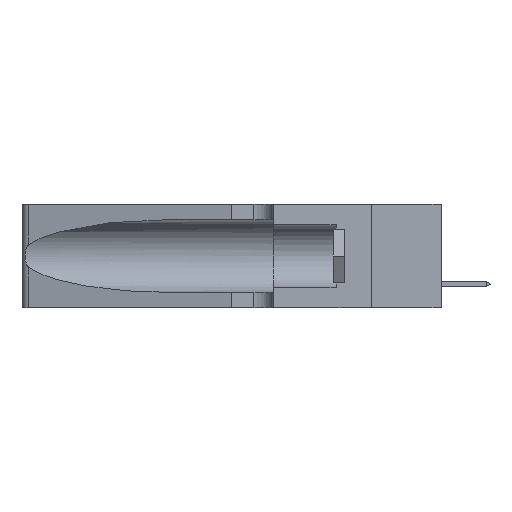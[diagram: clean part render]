
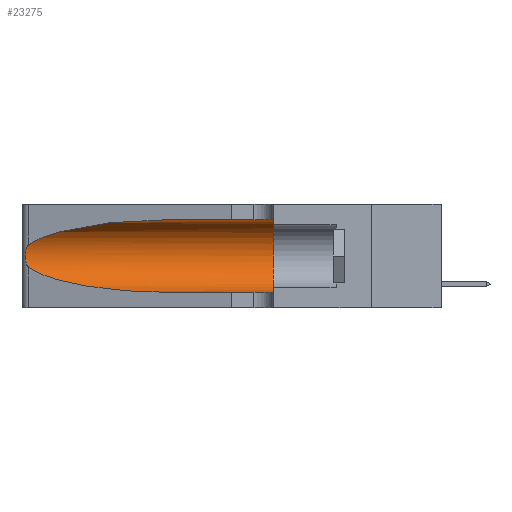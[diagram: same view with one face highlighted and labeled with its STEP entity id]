
A CAD part, left-side view. The second image highlights one B-rep face of the part: STEP entity #23275.
In plain terms, the highlighted cylindrical face has radius 3.308 mm (diameter 6.617 mm), a partial arc.
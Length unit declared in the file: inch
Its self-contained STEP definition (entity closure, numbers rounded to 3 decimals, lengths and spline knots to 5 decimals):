
#220 = CARTESIAN_POINT ( 'NONE',  ( 0.1305, 1.61858, 0.185 ) ) ;
#296 = CARTESIAN_POINT ( 'NONE',  ( 0.25555, 1.22993, 0.14849 ) ) ;
#635 = CIRCLE ( 'NONE', #13194, 0.13025 ) ;
#764 = CARTESIAN_POINT ( 'NONE',  ( 0.1305, 0.72297, 0.05475 ) ) ;
#858 = CARTESIAN_POINT ( 'NONE',  ( 0.1305, 0.72297, 0.31525 ) ) ;
#1042 = DIRECTION ( 'NONE',  ( 0., 0., 1. ) ) ;
#2047 = AXIS2_PLACEMENT_3D ( 'NONE', #220, #3992, #23539 ) ;
#2331 = CARTESIAN_POINT ( 'NONE',  ( 0.25639, 1.23186, 0.15144 ) ) ;
#2939 = VERTEX_POINT ( 'NONE', #21987 ) ;
#3081 = VECTOR ( 'NONE', #9644, 39.37008 ) ;
#3137 = LINE ( 'NONE', #10759, #8001 ) ;
#3707 = CYLINDRICAL_SURFACE ( 'NONE', #2047, 0.13025 ) ;
#3813 = VERTEX_POINT ( 'NONE', #22875 ) ;
#3992 = DIRECTION ( 'NONE',  ( 0., -1., 0. ) ) ;
#4366 = CARTESIAN_POINT ( 'NONE',  ( 0.25789, 1.23486, 0.15765 ) ) ;
#4526 = CARTESIAN_POINT ( 'NONE',  ( 0.2373, 1.15595, 0.08982 ) ) ;
#4982 = DIRECTION ( 'NONE',  ( 0., -1., 0. ) ) ;
#6987 = VERTEX_POINT ( 'NONE', #23021 ) ;
#7429 = ORIENTED_EDGE ( 'NONE', *, *, #23166, .T. ) ;
#7462 = CARTESIAN_POINT ( 'NONE',  ( 0.25487, 1.22718, 0.22369 ) ) ;
#7702 = CARTESIAN_POINT ( 'NONE',  ( 0.25555, 1.22994, 0.2215 ) ) ;
#8001 = VECTOR ( 'NONE', #4982, 39.37008 ) ;
#9298 = CARTESIAN_POINT ( 'NONE',  ( 0.1305, 1.61858, 0.05475 ) ) ;
#9644 = DIRECTION ( 'NONE',  ( 0., -1., 0. ) ) ;
#9649 = EDGE_CURVE ( 'NONE', #6987, #13313, #10922, .T. ) ;
#9994 = CARTESIAN_POINT ( 'NONE',  ( 0.25487, 1.22718, 0.22369 ) ) ;
#10265 = CARTESIAN_POINT ( 'NONE',  ( 0.25487, 1.22718, 0.14631 ) ) ;
#10544 = CARTESIAN_POINT ( 'NONE',  ( 0.25487, 1.22718, 0.14631 ) ) ;
#10554 = CARTESIAN_POINT ( 'NONE',  ( 0.26018, 1.23835, 0.19895 ) ) ;
#10759 = CARTESIAN_POINT ( 'NONE',  ( 0.1305, 1.61858, 0.31525 ) ) ;
#10922 = B_SPLINE_CURVE_WITH_KNOTS ( 'NONE', 3,
 ( #7462, #7702, #11607, #17518, #19937, #10554, #22678, #18509, #24903, #15710, #4366, #2331, #296, #10265 ),
 .UNSPECIFIED., .F., .F.,
 ( 4, 2, 2, 2, 2, 2, 4 ),
 ( 0., 0.00027, 0.00053, 0.00107, 0.0016, 0.00187, 0.00214 ),
 .UNSPECIFIED. ) ;
#11607 = CARTESIAN_POINT ( 'NONE',  ( 0.25639, 1.23184, 0.21858 ) ) ;
#11633 = CARTESIAN_POINT ( 'NONE',  ( 0.1305, 0.72297, 0.31525 ) ) ;
#11714 = CARTESIAN_POINT ( 'NONE',  ( 0.2373, 1.15595, 0.28018 ) ) ;
#11769 = ORIENTED_EDGE ( 'NONE', *, *, #22308, .F. ) ;
#12481 = CARTESIAN_POINT ( 'NONE',  ( 0.18966, 0.96281, 0.05475 ) ) ;
#12771 = CARTESIAN_POINT ( 'NONE',  ( 0.1305, 0.35, 0.185 ) ) ;
#12949 = DIRECTION ( 'NONE',  ( 0., 1., 0. ) ) ;
#13194 = AXIS2_PLACEMENT_3D ( 'NONE', #12771, #12949, #1042 ) ;
#13313 = VERTEX_POINT ( 'NONE', #10544 ) ;
#13550 = ORIENTED_EDGE ( 'NONE', *, *, #19743, .T. ) ;
#14144 = VERTEX_POINT ( 'NONE', #858 ) ;
#14718 = CARTESIAN_POINT ( 'NONE',  ( 0.25487, 1.22718, 0.14631 ) ) ;
#14924 = EDGE_CURVE ( 'NONE', #14144, #2939, #3137, .T. ) ;
#15461 = EDGE_LOOP ( 'NONE', ( #13550, #18067, #15546, #7429, #11769, #24897 ) ) ;
#15546 = ORIENTED_EDGE ( 'NONE', *, *, #18518, .T. ) ;
#15710 = CARTESIAN_POINT ( 'NONE',  ( 0.25856, 1.23593, 0.16098 ) ) ;
#16302 = VERTEX_POINT ( 'NONE', #20166 ) ;
#17518 = CARTESIAN_POINT ( 'NONE',  ( 0.25787, 1.23484, 0.2124 ) ) ;
#18067 = ORIENTED_EDGE ( 'NONE', *, *, #9649, .T. ) ;
#18132 =( BOUNDED_CURVE ( )  B_SPLINE_CURVE ( 3, ( #14718, #4526, #12481, #764 ),
 .UNSPECIFIED., .F., .T. ) 
 B_SPLINE_CURVE_WITH_KNOTS ( ( 4, 4 ),
 ( 3.44316, 4.71239 ),
 .UNSPECIFIED. ) 
 CURVE ( )  GEOMETRIC_REPRESENTATION_ITEM ( )  RATIONAL_B_SPLINE_CURVE ( ( 1., 0.87, 0.87, 1. ) ) 
 REPRESENTATION_ITEM ( '' )  );
#18509 = CARTESIAN_POINT ( 'NONE',  ( 0.26075, 1.23896, 0.178 ) ) ;
#18518 = EDGE_CURVE ( 'NONE', #13313, #3813, #18132, .T. ) ;
#19276 = FACE_OUTER_BOUND ( 'NONE', #15461, .T. ) ;
#19743 = EDGE_CURVE ( 'NONE', #14144, #6987, #22166, .T. ) ;
#19937 = CARTESIAN_POINT ( 'NONE',  ( 0.25854, 1.2359, 0.20912 ) ) ;
#20166 = CARTESIAN_POINT ( 'NONE',  ( 0.1305, 0.35, 0.05475 ) ) ;
#20760 = LINE ( 'NONE', #9298, #3081 ) ;
#21987 = CARTESIAN_POINT ( 'NONE',  ( 0.1305, 0.35, 0.31525 ) ) ;
#22166 =( BOUNDED_CURVE ( )  B_SPLINE_CURVE ( 3, ( #11633, #23506, #11714, #9994 ),
 .UNSPECIFIED., .F., .T. ) 
 B_SPLINE_CURVE_WITH_KNOTS ( ( 4, 4 ),
 ( 1.5708, 2.84003 ),
 .UNSPECIFIED. ) 
 CURVE ( )  GEOMETRIC_REPRESENTATION_ITEM ( )  RATIONAL_B_SPLINE_CURVE ( ( 1., 0.87, 0.87, 1. ) ) 
 REPRESENTATION_ITEM ( '' )  );
#22308 = EDGE_CURVE ( 'NONE', #2939, #16302, #635, .T. ) ;
#22678 = CARTESIAN_POINT ( 'NONE',  ( 0.26075, 1.23896, 0.19203 ) ) ;
#22875 = CARTESIAN_POINT ( 'NONE',  ( 0.1305, 0.72297, 0.05475 ) ) ;
#23021 = CARTESIAN_POINT ( 'NONE',  ( 0.25487, 1.22718, 0.22369 ) ) ;
#23166 = EDGE_CURVE ( 'NONE', #3813, #16302, #20760, .T. ) ;
#23275 = ADVANCED_FACE ( 'NONE', ( #19276 ), #3707, .F. ) ;
#23506 = CARTESIAN_POINT ( 'NONE',  ( 0.18966, 0.96281, 0.31525 ) ) ;
#23539 = DIRECTION ( 'NONE',  ( 0., 0., -1. ) ) ;
#24897 = ORIENTED_EDGE ( 'NONE', *, *, #14924, .F. ) ;
#24903 = CARTESIAN_POINT ( 'NONE',  ( 0.26017, 1.23833, 0.17102 ) ) ;
